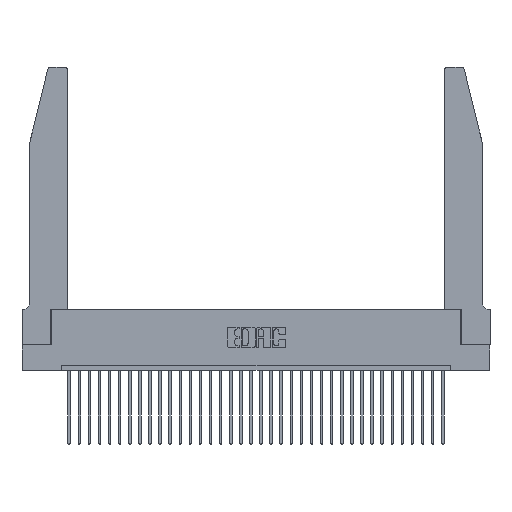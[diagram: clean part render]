
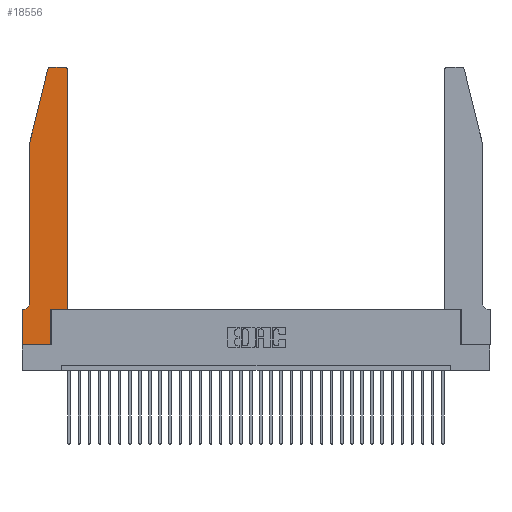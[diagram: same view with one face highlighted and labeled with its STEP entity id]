
A CAD part, top view. The second image highlights one B-rep face of the part: STEP entity #18556.
In plain terms, the highlighted planar face has unit normal (0, 0, 1).
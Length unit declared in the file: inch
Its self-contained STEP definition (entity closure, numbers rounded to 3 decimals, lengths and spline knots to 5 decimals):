
#65 = AXIS2_PLACEMENT_3D ( 'NONE', #22505, #17158, #1729 ) ;
#140 = VERTEX_POINT ( 'NONE', #16583 ) ;
#240 = DIRECTION ( 'NONE',  ( -0.239, -0.971, 0. ) ) ;
#721 = ORIENTED_EDGE ( 'NONE', *, *, #4046, .T. ) ;
#795 = ORIENTED_EDGE ( 'NONE', *, *, #28464, .T. ) ;
#992 = CARTESIAN_POINT ( 'NONE',  ( 0., 0.35, 0.37 ) ) ;
#1433 = DIRECTION ( 'NONE',  ( 0., 0., 1. ) ) ;
#1447 = PLANE ( 'NONE',  #14573 ) ;
#1729 = DIRECTION ( 'NONE',  ( -1., 0., 0. ) ) ;
#2529 = CIRCLE ( 'NONE', #8970, 0.03 ) ;
#2643 = CARTESIAN_POINT ( 'NONE',  ( 0.0755, 0.35, 0.37 ) ) ;
#2978 = VERTEX_POINT ( 'NONE', #7880 ) ;
#4046 = EDGE_CURVE ( 'NONE', #6988, #25182, #2529, .T. ) ;
#4056 = DIRECTION ( 'NONE',  ( 1., 0., 0. ) ) ;
#4923 = CARTESIAN_POINT ( 'NONE',  ( 0.25487, 2.72718, 0.37 ) ) ;
#5513 = LINE ( 'NONE', #15020, #25134 ) ;
#5928 = EDGE_CURVE ( 'NONE', #24343, #6988, #20492, .T. ) ;
#6018 = VECTOR ( 'NONE', #31763, 39.37008 ) ;
#6741 = LINE ( 'NONE', #33524, #14119 ) ;
#6988 = VERTEX_POINT ( 'NONE', #32886 ) ;
#7224 = DIRECTION ( 'NONE',  ( 1., 0., 0. ) ) ;
#7425 = CARTESIAN_POINT ( 'NONE',  ( 0.0055, 0.35, 0.37 ) ) ;
#7652 = LINE ( 'NONE', #32312, #15786 ) ;
#7880 = CARTESIAN_POINT ( 'NONE',  ( 0., 0., 0.37 ) ) ;
#7896 = EDGE_CURVE ( 'NONE', #30478, #8988, #13011, .T. ) ;
#8970 = AXIS2_PLACEMENT_3D ( 'NONE', #22845, #20671, #7224 ) ;
#8988 = VERTEX_POINT ( 'NONE', #7425 ) ;
#9320 = LINE ( 'NONE', #26854, #30588 ) ;
#9859 = ORIENTED_EDGE ( 'NONE', *, *, #13901, .T. ) ;
#10325 = EDGE_CURVE ( 'NONE', #22076, #30478, #5513, .T. ) ;
#10623 = VECTOR ( 'NONE', #14352, 39.37008 ) ;
#11126 = EDGE_CURVE ( 'NONE', #20408, #26689, #18119, .T. ) ;
#12110 = CARTESIAN_POINT ( 'NONE',  ( 0., 0.35, 0.37 ) ) ;
#12368 = ORIENTED_EDGE ( 'NONE', *, *, #28676, .T. ) ;
#12449 = ORIENTED_EDGE ( 'NONE', *, *, #26073, .T. ) ;
#12881 = DIRECTION ( 'NONE',  ( 1., 0., 0. ) ) ;
#13011 = CIRCLE ( 'NONE', #65, 0.07 ) ;
#13505 = CIRCLE ( 'NONE', #32604, 0.03 ) ;
#13901 = EDGE_CURVE ( 'NONE', #26689, #24343, #6741, .T. ) ;
#14119 = VECTOR ( 'NONE', #12881, 39.37008 ) ;
#14352 = DIRECTION ( 'NONE',  ( 1., 0., 0. ) ) ;
#14489 = CARTESIAN_POINT ( 'NONE',  ( 0.284, 2.72, 0.37 ) ) ;
#14573 = AXIS2_PLACEMENT_3D ( 'NONE', #12110, #30245, #25375 ) ;
#15020 = CARTESIAN_POINT ( 'NONE',  ( 0.0755, 2., 0.37 ) ) ;
#15134 = DIRECTION ( 'NONE',  ( 0., -1., 0. ) ) ;
#15786 = VECTOR ( 'NONE', #16688, 39.37008 ) ;
#16583 = CARTESIAN_POINT ( 'NONE',  ( 0.284, 2.75, 0.37 ) ) ;
#16688 = DIRECTION ( 'NONE',  ( -1., 0., 0. ) ) ;
#16819 = VERTEX_POINT ( 'NONE', #992 ) ;
#17158 = DIRECTION ( 'NONE',  ( 0., 0., -1. ) ) ;
#17357 = CARTESIAN_POINT ( 'NONE',  ( 0.4205, 2.75, 0.37 ) ) ;
#17651 = VECTOR ( 'NONE', #27154, 39.37008 ) ;
#18119 = LINE ( 'NONE', #26437, #23399 ) ;
#18463 = ORIENTED_EDGE ( 'NONE', *, *, #5928, .T. ) ;
#18556 = ADVANCED_FACE ( 'NONE', ( #30896 ), #1447, .T. ) ;
#18608 = DIRECTION ( 'NONE',  ( 0., -1., 0. ) ) ;
#18611 = CARTESIAN_POINT ( 'NONE',  ( 0.0755, 0.42, 0.37 ) ) ;
#18810 = ORIENTED_EDGE ( 'NONE', *, *, #29592, .T. ) ;
#20408 = VERTEX_POINT ( 'NONE', #32359 ) ;
#20492 = LINE ( 'NONE', #24641, #17651 ) ;
#20513 = CARTESIAN_POINT ( 'NONE',  ( 0.2865, 0.35, 0.37 ) ) ;
#20671 = DIRECTION ( 'NONE',  ( 0., 0., 1. ) ) ;
#21136 = ORIENTED_EDGE ( 'NONE', *, *, #22329, .T. ) ;
#21908 = ORIENTED_EDGE ( 'NONE', *, *, #11126, .T. ) ;
#22076 = VERTEX_POINT ( 'NONE', #27150 ) ;
#22329 = EDGE_CURVE ( 'NONE', #2978, #20408, #28976, .T. ) ;
#22505 = CARTESIAN_POINT ( 'NONE',  ( 0.0055, 0.42, 0.37 ) ) ;
#22657 = VECTOR ( 'NONE', #240, 39.37008 ) ;
#22845 = CARTESIAN_POINT ( 'NONE',  ( 0.4205, 2.72, 0.37 ) ) ;
#23399 = VECTOR ( 'NONE', #23666, 39.37008 ) ;
#23604 = VERTEX_POINT ( 'NONE', #4923 ) ;
#23666 = DIRECTION ( 'NONE',  ( 0., 1., 0. ) ) ;
#24302 = LINE ( 'NONE', #28991, #22657 ) ;
#24343 = VERTEX_POINT ( 'NONE', #24927 ) ;
#24641 = CARTESIAN_POINT ( 'NONE',  ( 0.4505, 0.35, 0.37 ) ) ;
#24927 = CARTESIAN_POINT ( 'NONE',  ( 0.4505, 0.35, 0.37 ) ) ;
#25134 = VECTOR ( 'NONE', #15134, 39.37008 ) ;
#25182 = VERTEX_POINT ( 'NONE', #17357 ) ;
#25244 = ORIENTED_EDGE ( 'NONE', *, *, #10325, .T. ) ;
#25264 = LINE ( 'NONE', #2643, #6018 ) ;
#25375 = DIRECTION ( 'NONE',  ( 1., 0., 0. ) ) ;
#26073 = EDGE_CURVE ( 'NONE', #140, #23604, #13505, .T. ) ;
#26437 = CARTESIAN_POINT ( 'NONE',  ( 0.2865, 0.35, 0.37 ) ) ;
#26689 = VERTEX_POINT ( 'NONE', #20513 ) ;
#26854 = CARTESIAN_POINT ( 'NONE',  ( 0., 0., 0.37 ) ) ;
#27145 = CARTESIAN_POINT ( 'NONE',  ( 0., 0., 0.37 ) ) ;
#27150 = CARTESIAN_POINT ( 'NONE',  ( 0.0755, 2., 0.37 ) ) ;
#27154 = DIRECTION ( 'NONE',  ( 0., 1., 0. ) ) ;
#27208 = EDGE_CURVE ( 'NONE', #16819, #2978, #9320, .T. ) ;
#28464 = EDGE_CURVE ( 'NONE', #8988, #16819, #25264, .T. ) ;
#28633 = ORIENTED_EDGE ( 'NONE', *, *, #7896, .T. ) ;
#28654 = ORIENTED_EDGE ( 'NONE', *, *, #27208, .T. ) ;
#28676 = EDGE_CURVE ( 'NONE', #25182, #140, #7652, .T. ) ;
#28976 = LINE ( 'NONE', #27145, #10623 ) ;
#28991 = CARTESIAN_POINT ( 'NONE',  ( 0.0755, 2., 0.37 ) ) ;
#29592 = EDGE_CURVE ( 'NONE', #23604, #22076, #24302, .T. ) ;
#30245 = DIRECTION ( 'NONE',  ( 0., 0., 1. ) ) ;
#30478 = VERTEX_POINT ( 'NONE', #18611 ) ;
#30588 = VECTOR ( 'NONE', #18608, 39.37008 ) ;
#30750 = EDGE_LOOP ( 'NONE', ( #12368, #12449, #18810, #25244, #28633, #795, #28654, #21136, #21908, #9859, #18463, #721 ) ) ;
#30896 = FACE_OUTER_BOUND ( 'NONE', #30750, .T. ) ;
#31763 = DIRECTION ( 'NONE',  ( -1., 0., 0. ) ) ;
#32312 = CARTESIAN_POINT ( 'NONE',  ( 0.2605, 2.75, 0.37 ) ) ;
#32359 = CARTESIAN_POINT ( 'NONE',  ( 0.2865, 0., 0.37 ) ) ;
#32604 = AXIS2_PLACEMENT_3D ( 'NONE', #14489, #1433, #4056 ) ;
#32886 = CARTESIAN_POINT ( 'NONE',  ( 0.4505, 2.72, 0.37 ) ) ;
#33524 = CARTESIAN_POINT ( 'NONE',  ( 0.4505, 0.35, 0.37 ) ) ;
